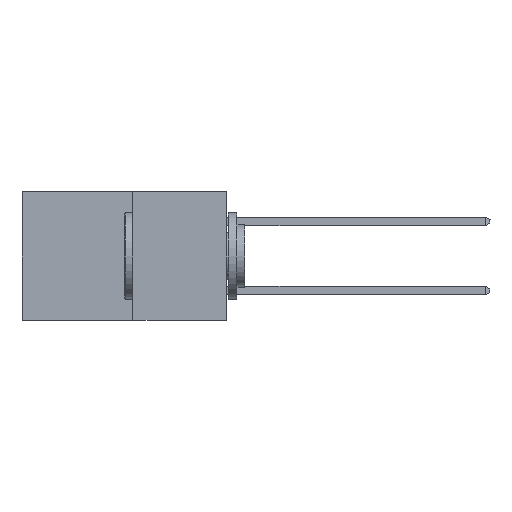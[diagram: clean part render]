
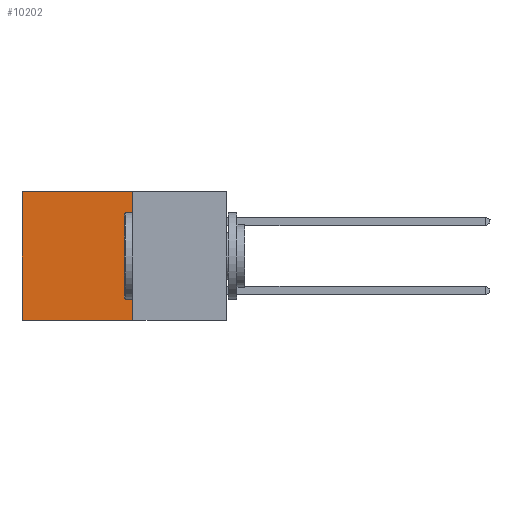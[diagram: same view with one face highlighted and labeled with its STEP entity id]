
A CAD part, left-side view. The second image highlights one B-rep face of the part: STEP entity #10202.
In plain terms, the highlighted planar face has unit normal (-1, 0, 0).
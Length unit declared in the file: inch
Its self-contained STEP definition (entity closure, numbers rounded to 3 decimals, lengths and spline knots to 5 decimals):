
#45 = LINE ( 'NONE', #26583, #29388 ) ;
#2231 = AXIS2_PLACEMENT_3D ( 'NONE', #25104, #6623, #29657 ) ;
#3253 = LINE ( 'NONE', #27881, #9613 ) ;
#3484 = DIRECTION ( 'NONE',  ( 0., 0., -1. ) ) ;
#3607 = VERTEX_POINT ( 'NONE', #27945 ) ;
#4879 = DIRECTION ( 'NONE',  ( 0., 1., 0. ) ) ;
#5404 = DIRECTION ( 'NONE',  ( 0., 0., -1. ) ) ;
#5509 = CARTESIAN_POINT ( 'NONE',  ( 0.277, 0.27, 0. ) ) ;
#5584 = CARTESIAN_POINT ( 'NONE',  ( 0.277, 0.59, -0.37 ) ) ;
#5720 = CARTESIAN_POINT ( 'NONE',  ( 0.277, 0.27, -0.37 ) ) ;
#5730 = FACE_OUTER_BOUND ( 'NONE', #24414, .T. ) ;
#6623 = DIRECTION ( 'NONE',  ( 1., 0., 0. ) ) ;
#6666 = EDGE_CURVE ( 'NONE', #24102, #3607, #24354, .T. ) ;
#7500 = ORIENTED_EDGE ( 'NONE', *, *, #17791, .F. ) ;
#7913 = ORIENTED_EDGE ( 'NONE', *, *, #26448, .F. ) ;
#9613 = VECTOR ( 'NONE', #4879, 39.37008 ) ;
#10202 = ADVANCED_FACE ( 'NONE', ( #5730 ), #27399, .F. ) ;
#10388 = EDGE_CURVE ( 'NONE', #23706, #24102, #24535, .T. ) ;
#10731 = VECTOR ( 'NONE', #5404, 39.37008 ) ;
#13095 = ORIENTED_EDGE ( 'NONE', *, *, #6666, .T. ) ;
#13974 = CARTESIAN_POINT ( 'NONE',  ( 0.277, 0.59, 0. ) ) ;
#14269 = ORIENTED_EDGE ( 'NONE', *, *, #10388, .T. ) ;
#17791 = EDGE_CURVE ( 'NONE', #28250, #3607, #3253, .T. ) ;
#18503 = VECTOR ( 'NONE', #23488, 39.37008 ) ;
#21215 = CARTESIAN_POINT ( 'NONE',  ( 0.277, 0.27, 0. ) ) ;
#23488 = DIRECTION ( 'NONE',  ( 0., 1., 0. ) ) ;
#23706 = VERTEX_POINT ( 'NONE', #5509 ) ;
#24102 = VERTEX_POINT ( 'NONE', #13974 ) ;
#24354 = LINE ( 'NONE', #5584, #10731 ) ;
#24414 = EDGE_LOOP ( 'NONE', ( #13095, #7500, #7913, #14269 ) ) ;
#24535 = LINE ( 'NONE', #21215, #18503 ) ;
#25104 = CARTESIAN_POINT ( 'NONE',  ( 0.277, 0.27, -0.37 ) ) ;
#26448 = EDGE_CURVE ( 'NONE', #23706, #28250, #45, .T. ) ;
#26583 = CARTESIAN_POINT ( 'NONE',  ( 0.277, 0.27, -0.37 ) ) ;
#27399 = PLANE ( 'NONE',  #2231 ) ;
#27881 = CARTESIAN_POINT ( 'NONE',  ( 0.277, 0.27, -0.37 ) ) ;
#27945 = CARTESIAN_POINT ( 'NONE',  ( 0.277, 0.59, -0.37 ) ) ;
#28250 = VERTEX_POINT ( 'NONE', #5720 ) ;
#29388 = VECTOR ( 'NONE', #3484, 39.37008 ) ;
#29657 = DIRECTION ( 'NONE',  ( 0., 0., -1. ) ) ;
